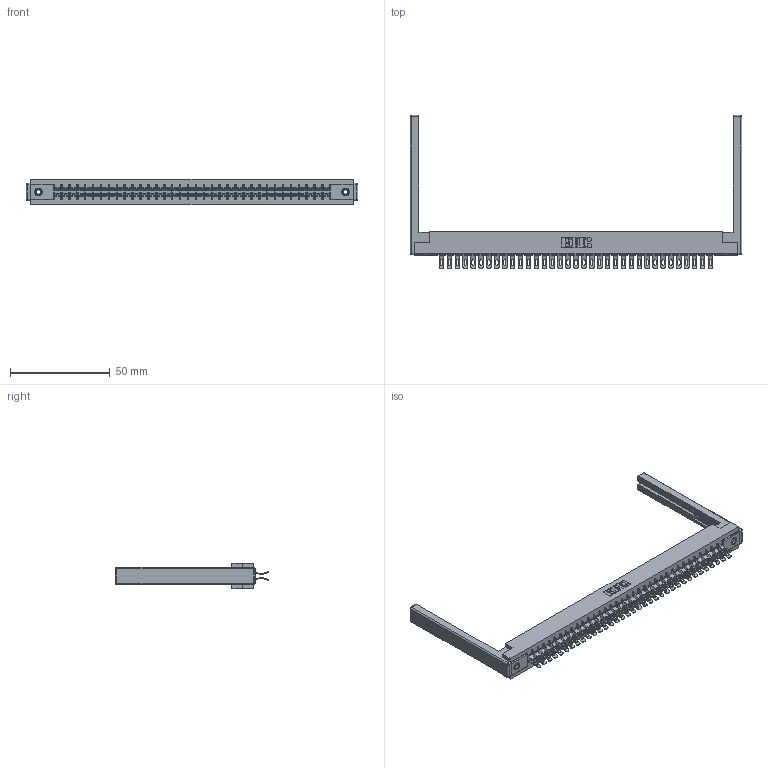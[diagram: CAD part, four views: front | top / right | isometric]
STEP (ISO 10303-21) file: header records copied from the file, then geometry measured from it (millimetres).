
FILE_DESCRIPTION (( 'STEP AP203' ), '1' );
FILE_NAME ('355-070-555-268.STEP', '2019-09-12T17:38:16', ( '' ), ( '' ), 'SwSTEP 2.0', 'SolidWorks 2016', '' );
FILE_SCHEMA (( 'CONFIG_CONTROL_DESIGN' ));
Length unit declared in the file: inch
Products named in the file (5): 345-250-001_345-250-001-102; 307-220-068; 355-070-555-268; 305 Part_.156 Dia; 305-290-001_555
Assembly tree (75 placements, depth 2):
  355-070-555-268
    305 Part_.156 Dia
    305-290-001_555  x70
    345-250-001_345-250-001-102  x2
    307-220-068  x2
Bounding box: 166.12 x 76.71 x 12.7 mm (x, y, z)
Volume: 21878.8 mm3; surface area: 27388.9 mm2
Topology: 75 solids, 75 shells, 4890 faces, 14531 edges, 9478 vertices
Faces by surface type: plane 2396, cylinder 2330, sphere 148, cone 12, torus 4
Entity records: 42131 total; most frequent: CARTESIAN_POINT 6962, ORIENTED_EDGE 6892, DIRECTION 6754, EDGE_CURVE 3446, LINE 2750, VECTOR 2750, VERTEX_POINT 2194, AXIS2_PLACEMENT_3D 2002
